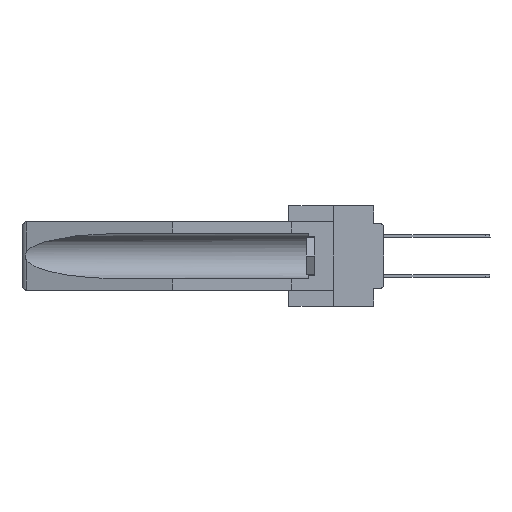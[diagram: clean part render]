
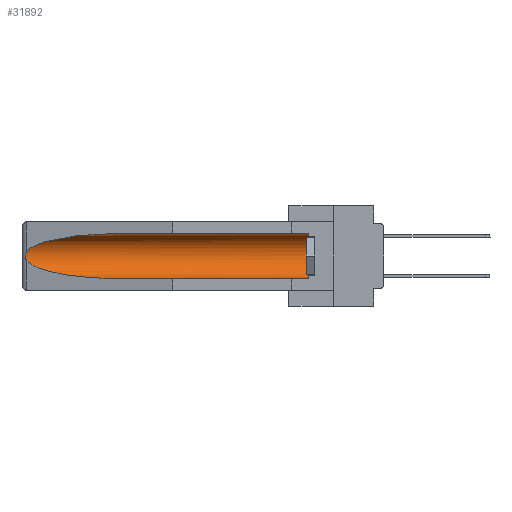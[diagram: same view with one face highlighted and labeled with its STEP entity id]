
A CAD part, left-side view. The second image highlights one B-rep face of the part: STEP entity #31892.
In plain terms, the highlighted cylindrical face has radius 2.857 mm (diameter 5.715 mm), a partial arc.
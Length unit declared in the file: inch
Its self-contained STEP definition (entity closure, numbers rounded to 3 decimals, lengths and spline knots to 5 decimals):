
#144 = B_SPLINE_CURVE_WITH_KNOTS ( 'NONE', 3,
 ( #33518, #539, #21398, #18362, #36635, #9542, #27569, #36772, #12190, #9294 ),
 .UNSPECIFIED., .F., .F.,
 ( 4, 2, 2, 2, 4 ),
 ( 0., 0.00029, 0.00058, 0.00087, 0.00117 ),
 .UNSPECIFIED. ) ;
#539 = CARTESIAN_POINT ( 'NONE',  ( 0.26597, 1.52961, -0.15275 ) ) ;
#673 = CYLINDRICAL_SURFACE ( 'NONE', #7453, 0.1125 ) ;
#1958 = CARTESIAN_POINT ( 'NONE',  ( 0.25451, 1.48313, -0.09465 ) ) ;
#3135 = DIRECTION ( 'NONE',  ( 0., 1., 0. ) ) ;
#3352 = DIRECTION ( 'NONE',  ( 0., 1., 0. ) ) ;
#3389 = CARTESIAN_POINT ( 'NONE',  ( 0.155, -0.30754, -0.059 ) ) ;
#5233 = CARTESIAN_POINT ( 'NONE',  ( 0.26537, 1.52718, -0.14972 ) ) ;
#5310 =( BOUNDED_CURVE ( )  B_SPLINE_CURVE ( 3, ( #38266, #29214, #1958, #8175 ),
 .UNSPECIFIED., .F., .F. ) 
 B_SPLINE_CURVE_WITH_KNOTS ( ( 4, 4 ),
 ( 4.71239, 6.08839 ),
 .UNSPECIFIED. ) 
 CURVE ( )  GEOMETRIC_REPRESENTATION_ITEM ( )  RATIONAL_B_SPLINE_CURVE ( ( 1., 0.848, 0.848, 1. ) ) 
 REPRESENTATION_ITEM ( '' )  );
#5416 = EDGE_CURVE ( 'NONE', #29149, #7016, #144, .T. ) ;
#5455 = CARTESIAN_POINT ( 'NONE',  ( 0.21114, 1.30732, -0.284 ) ) ;
#5479 = CARTESIAN_POINT ( 'NONE',  ( 0.155, -0.30754, -0.1715 ) ) ;
#7016 = VERTEX_POINT ( 'NONE', #26683 ) ;
#7281 = AXIS2_PLACEMENT_3D ( 'NONE', #38317, #14654, #11356 ) ;
#7354 = EDGE_CURVE ( 'NONE', #24874, #16811, #34442, .T. ) ;
#7453 = AXIS2_PLACEMENT_3D ( 'NONE', #5479, #29570, #8258 ) ;
#8175 = CARTESIAN_POINT ( 'NONE',  ( 0.26537, 1.52718, -0.14972 ) ) ;
#8258 = DIRECTION ( 'NONE',  ( 0., 0., 1. ) ) ;
#8872 = CARTESIAN_POINT ( 'NONE',  ( 0.25451, 1.48313, -0.24835 ) ) ;
#9294 = CARTESIAN_POINT ( 'NONE',  ( 0.26537, 1.52718, -0.19328 ) ) ;
#9542 = CARTESIAN_POINT ( 'NONE',  ( 0.2675, 1.53308, -0.17534 ) ) ;
#10092 = ORIENTED_EDGE ( 'NONE', *, *, #15771, .T. ) ;
#11356 = DIRECTION ( 'NONE',  ( 0., 0., 1. ) ) ;
#12190 = CARTESIAN_POINT ( 'NONE',  ( 0.26597, 1.5296, -0.19026 ) ) ;
#13322 = CARTESIAN_POINT ( 'NONE',  ( 0.155, 0.126, -0.284 ) ) ;
#14502 = CIRCLE ( 'NONE', #7281, 0.1125 ) ;
#14528 = CARTESIAN_POINT ( 'NONE',  ( 0.155, 1.07973, -0.284 ) ) ;
#14540 = ORIENTED_EDGE ( 'NONE', *, *, #25117, .T. ) ;
#14654 = DIRECTION ( 'NONE',  ( 0., -1., 0. ) ) ;
#15771 = EDGE_CURVE ( 'NONE', #27522, #29149, #5310, .T. ) ;
#16158 = ORIENTED_EDGE ( 'NONE', *, *, #25800, .T. ) ;
#16811 = VERTEX_POINT ( 'NONE', #35424 ) ;
#18362 = CARTESIAN_POINT ( 'NONE',  ( 0.2673, 1.5327, -0.16383 ) ) ;
#20015 =( BOUNDED_CURVE ( )  B_SPLINE_CURVE ( 3, ( #29536, #8872, #5455, #14528 ),
 .UNSPECIFIED., .F., .F. ) 
 B_SPLINE_CURVE_WITH_KNOTS ( ( 4, 4 ),
 ( 0.1948, 1.5708 ),
 .UNSPECIFIED. ) 
 CURVE ( )  GEOMETRIC_REPRESENTATION_ITEM ( )  RATIONAL_B_SPLINE_CURVE ( ( 1., 0.848, 0.848, 1. ) ) 
 REPRESENTATION_ITEM ( '' )  );
#20382 = ORIENTED_EDGE ( 'NONE', *, *, #7354, .F. ) ;
#21398 = CARTESIAN_POINT ( 'NONE',  ( 0.26654, 1.53092, -0.15636 ) ) ;
#22964 = ORIENTED_EDGE ( 'NONE', *, *, #35842, .T. ) ;
#24319 = LINE ( 'NONE', #3389, #31860 ) ;
#24874 = VERTEX_POINT ( 'NONE', #13322 ) ;
#25117 = EDGE_CURVE ( 'NONE', #24874, #37372, #14502, .T. ) ;
#25478 = CARTESIAN_POINT ( 'NONE',  ( 0.155, -0.30754, -0.284 ) ) ;
#25800 = EDGE_CURVE ( 'NONE', #37372, #27522, #24319, .T. ) ;
#26425 = VECTOR ( 'NONE', #3352, 39.37008 ) ;
#26683 = CARTESIAN_POINT ( 'NONE',  ( 0.26537, 1.52718, -0.19328 ) ) ;
#27522 = VERTEX_POINT ( 'NONE', #34634 ) ;
#27569 = CARTESIAN_POINT ( 'NONE',  ( 0.2673, 1.53269, -0.17917 ) ) ;
#29149 = VERTEX_POINT ( 'NONE', #5233 ) ;
#29214 = CARTESIAN_POINT ( 'NONE',  ( 0.21114, 1.30732, -0.059 ) ) ;
#29423 = ORIENTED_EDGE ( 'NONE', *, *, #5416, .T. ) ;
#29536 = CARTESIAN_POINT ( 'NONE',  ( 0.26537, 1.52718, -0.19328 ) ) ;
#29570 = DIRECTION ( 'NONE',  ( 0., 1., 0. ) ) ;
#29972 = FACE_OUTER_BOUND ( 'NONE', #30997, .T. ) ;
#30897 = CARTESIAN_POINT ( 'NONE',  ( 0.155, 0.126, -0.059 ) ) ;
#30997 = EDGE_LOOP ( 'NONE', ( #10092, #29423, #22964, #20382, #14540, #16158 ) ) ;
#31860 = VECTOR ( 'NONE', #3135, 39.37008 ) ;
#31892 = ADVANCED_FACE ( 'NONE', ( #29972 ), #673, .F. ) ;
#33518 = CARTESIAN_POINT ( 'NONE',  ( 0.26537, 1.52718, -0.14972 ) ) ;
#34442 = LINE ( 'NONE', #25478, #26425 ) ;
#34634 = CARTESIAN_POINT ( 'NONE',  ( 0.155, 1.07973, -0.059 ) ) ;
#35424 = CARTESIAN_POINT ( 'NONE',  ( 0.155, 1.07973, -0.284 ) ) ;
#35842 = EDGE_CURVE ( 'NONE', #7016, #16811, #20015, .T. ) ;
#36635 = CARTESIAN_POINT ( 'NONE',  ( 0.2675, 1.53308, -0.16763 ) ) ;
#36772 = CARTESIAN_POINT ( 'NONE',  ( 0.26655, 1.53094, -0.18657 ) ) ;
#37372 = VERTEX_POINT ( 'NONE', #30897 ) ;
#38266 = CARTESIAN_POINT ( 'NONE',  ( 0.155, 1.07973, -0.059 ) ) ;
#38317 = CARTESIAN_POINT ( 'NONE',  ( 0.155, 0.126, -0.1715 ) ) ;
